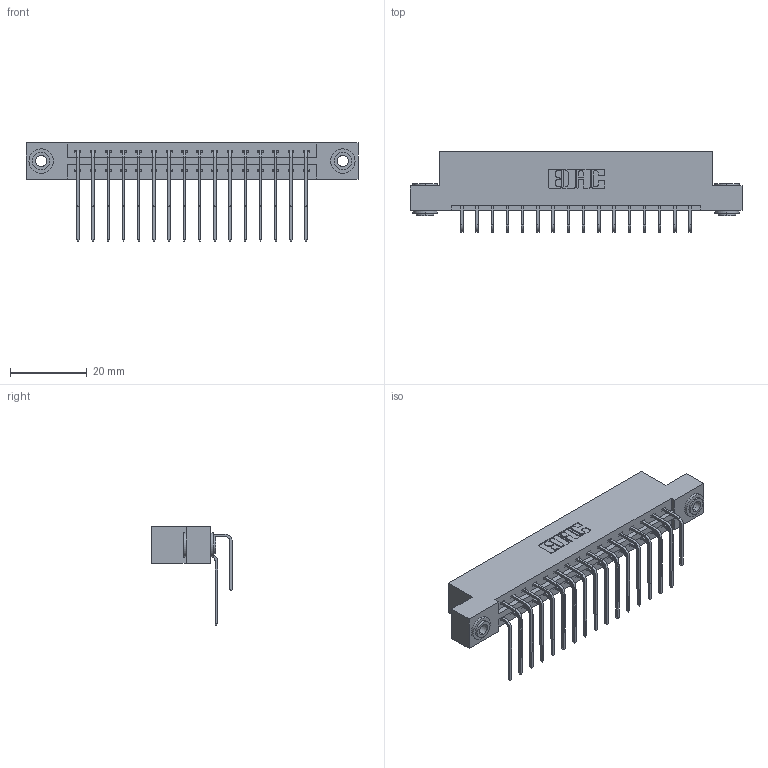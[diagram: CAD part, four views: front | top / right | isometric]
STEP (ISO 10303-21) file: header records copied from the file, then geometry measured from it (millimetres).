
FILE_DESCRIPTION (( 'STEP AP203' ), '1' );
FILE_NAME ('337-032-559-203.STEP', '2019-10-08T19:42:09', ( '' ), ( '' ), 'SwSTEP 2.0', 'SolidWorks 2016', '' );
FILE_SCHEMA (( 'CONFIG_CONTROL_DESIGN' ));
Length unit declared in the file: inch
Products named in the file (5): 337-032-559-203; 345-250-002_345-250-002-102; 337 Part_Flush Mounting Lugs - 0.156 Dia-TH; 345-292-001_558 559 Tail - 1; 345-292-001_559 Tail - 2
Assembly tree (35 placements, depth 2):
  337-032-559-203
    337 Part_Flush Mounting Lugs - 0.156 Dia-TH
    345-292-001_558 559 Tail - 1  x16
    345-292-001_559 Tail - 2  x16
    345-250-002_345-250-002-102  x2
Bounding box: 86.41 x 20.9 x 25.53 mm (x, y, z)
Volume: 8964.6 mm3; surface area: 11033.2 mm2
Topology: 35 solids, 35 shells, 1944 faces, 5731 edges, 3774 vertices
Faces by surface type: plane 1360, cylinder 576, cone 8
Entity records: 18202 total; most frequent: CARTESIAN_POINT 3108, ORIENTED_EDGE 2986, DIRECTION 2707, EDGE_CURVE 1493, LINE 1301, VECTOR 1301, VERTEX_POINT 990, AXIS2_PLACEMENT_3D 703
